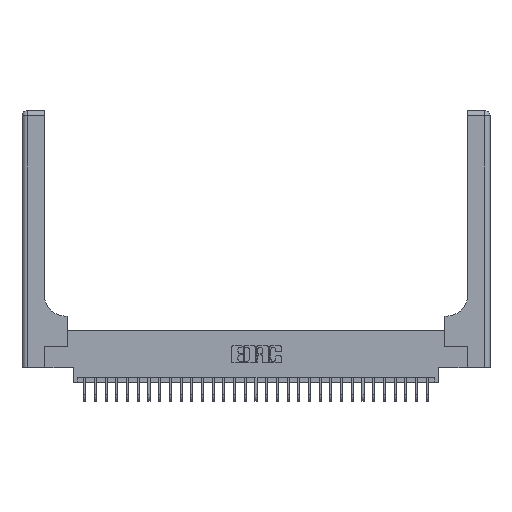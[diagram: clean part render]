
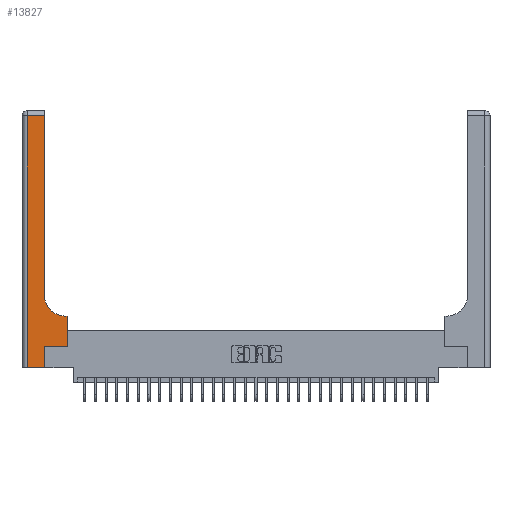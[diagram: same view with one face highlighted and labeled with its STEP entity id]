
A CAD part, top view. The second image highlights one B-rep face of the part: STEP entity #13827.
In plain terms, the highlighted planar face has unit normal (0, 0, 1).
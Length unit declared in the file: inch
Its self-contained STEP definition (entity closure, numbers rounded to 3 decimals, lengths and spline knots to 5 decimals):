
#315 = DIRECTION ( 'NONE',  ( 0., 1., 0. ) ) ;
#471 = CARTESIAN_POINT ( 'NONE',  ( 0.528, 0.25, 0.37 ) ) ;
#1172 = EDGE_CURVE ( 'NONE', #22529, #27195, #14642, .T. ) ;
#1348 = EDGE_CURVE ( 'NONE', #7076, #21148, #24732, .T. ) ;
#1525 = CARTESIAN_POINT ( 'NONE',  ( 0.06, 2.94, 0.37 ) ) ;
#1708 = CARTESIAN_POINT ( 'NONE',  ( 0.265, 0.25, 0.37 ) ) ;
#1849 = CARTESIAN_POINT ( 'NONE',  ( 0.265, 0.25, 0.37 ) ) ;
#2572 = VERTEX_POINT ( 'NONE', #21076 ) ;
#2679 = DIRECTION ( 'NONE',  ( 0., 0., -1. ) ) ;
#3170 = CARTESIAN_POINT ( 'NONE',  ( 0.06, 0., 0.37 ) ) ;
#3246 = AXIS2_PLACEMENT_3D ( 'NONE', #16298, #2679, #21384 ) ;
#4025 = EDGE_CURVE ( 'NONE', #10255, #10194, #4784, .T. ) ;
#4306 = ORIENTED_EDGE ( 'NONE', *, *, #1348, .T. ) ;
#4591 = EDGE_CURVE ( 'NONE', #10247, #22529, #27288, .T. ) ;
#4784 = LINE ( 'NONE', #16699, #14586 ) ;
#5008 = CARTESIAN_POINT ( 'NONE',  ( 0.265, 0., 0.37 ) ) ;
#5709 = DIRECTION ( 'NONE',  ( 1., 0., 0. ) ) ;
#5772 = CARTESIAN_POINT ( 'NONE',  ( 0.51, 0.6, 0.37 ) ) ;
#6225 = LINE ( 'NONE', #15553, #24726 ) ;
#7023 = ORIENTED_EDGE ( 'NONE', *, *, #20876, .T. ) ;
#7076 = VERTEX_POINT ( 'NONE', #27183 ) ;
#8366 = ORIENTED_EDGE ( 'NONE', *, *, #10621, .T. ) ;
#8431 = DIRECTION ( 'NONE',  ( 1., 0., 0. ) ) ;
#9112 = DIRECTION ( 'NONE',  ( -1., 0., 0. ) ) ;
#9415 = FACE_OUTER_BOUND ( 'NONE', #29696, .T. ) ;
#9507 = LINE ( 'NONE', #471, #24153 ) ;
#9653 = DIRECTION ( 'NONE',  ( -1., 0., 0. ) ) ;
#9687 = VECTOR ( 'NONE', #10799, 39.37008 ) ;
#10194 = VERTEX_POINT ( 'NONE', #5772 ) ;
#10247 = VERTEX_POINT ( 'NONE', #3170 ) ;
#10255 = VERTEX_POINT ( 'NONE', #29217 ) ;
#10621 = EDGE_CURVE ( 'NONE', #10194, #12486, #13497, .T. ) ;
#10799 = DIRECTION ( 'NONE',  ( 0., -1., 0. ) ) ;
#10882 = LINE ( 'NONE', #1708, #29936 ) ;
#10944 = CARTESIAN_POINT ( 'NONE',  ( 0.26, 0.85, 0.37 ) ) ;
#11467 = CARTESIAN_POINT ( 'NONE',  ( 0.265, 0., 0.37 ) ) ;
#12486 = VERTEX_POINT ( 'NONE', #10944 ) ;
#12857 = ORIENTED_EDGE ( 'NONE', *, *, #15804, .T. ) ;
#13141 = DIRECTION ( 'NONE',  ( 0., 0., -1. ) ) ;
#13228 = DIRECTION ( 'NONE',  ( -1., 0., 0. ) ) ;
#13292 = ORIENTED_EDGE ( 'NONE', *, *, #24489, .T. ) ;
#13402 = DIRECTION ( 'NONE',  ( 0., 1., 0. ) ) ;
#13497 = CIRCLE ( 'NONE', #3246, 0.25 ) ;
#13827 = ADVANCED_FACE ( 'NONE', ( #9415 ), #28128, .F. ) ;
#14586 = VECTOR ( 'NONE', #9653, 39.37008 ) ;
#14642 = LINE ( 'NONE', #5008, #27295 ) ;
#15553 = CARTESIAN_POINT ( 'NONE',  ( 0.26, 3., 0.37 ) ) ;
#15804 = EDGE_CURVE ( 'NONE', #27195, #2572, #10882, .T. ) ;
#16298 = CARTESIAN_POINT ( 'NONE',  ( 0.51, 0.85, 0.37 ) ) ;
#16699 = CARTESIAN_POINT ( 'NONE',  ( 0.26, 0.6, 0.37 ) ) ;
#17931 = EDGE_CURVE ( 'NONE', #21148, #10247, #29521, .T. ) ;
#18008 = VECTOR ( 'NONE', #8431, 39.37008 ) ;
#19139 = ORIENTED_EDGE ( 'NONE', *, *, #1172, .T. ) ;
#19397 = DIRECTION ( 'NONE',  ( 0., 1., 0. ) ) ;
#20308 = CARTESIAN_POINT ( 'NONE',  ( 0., 2.94, 0.37 ) ) ;
#20876 = EDGE_CURVE ( 'NONE', #2572, #10255, #9507, .T. ) ;
#21076 = CARTESIAN_POINT ( 'NONE',  ( 0.528, 0.25, 0.37 ) ) ;
#21148 = VERTEX_POINT ( 'NONE', #1525 ) ;
#21384 = DIRECTION ( 'NONE',  ( 1., 0., 0. ) ) ;
#21888 = ORIENTED_EDGE ( 'NONE', *, *, #4025, .T. ) ;
#22395 = CARTESIAN_POINT ( 'NONE',  ( 0., 0., 0.37 ) ) ;
#22479 = CARTESIAN_POINT ( 'NONE',  ( 0.06, 3., 0.37 ) ) ;
#22529 = VERTEX_POINT ( 'NONE', #11467 ) ;
#24153 = VECTOR ( 'NONE', #315, 39.37008 ) ;
#24287 = ORIENTED_EDGE ( 'NONE', *, *, #17931, .T. ) ;
#24489 = EDGE_CURVE ( 'NONE', #12486, #7076, #6225, .T. ) ;
#24726 = VECTOR ( 'NONE', #13402, 39.37008 ) ;
#24727 = AXIS2_PLACEMENT_3D ( 'NONE', #25826, #13141, #9112 ) ;
#24732 = LINE ( 'NONE', #20308, #28299 ) ;
#25826 = CARTESIAN_POINT ( 'NONE',  ( 0., 3., 0.37 ) ) ;
#27183 = CARTESIAN_POINT ( 'NONE',  ( 0.26, 2.94, 0.37 ) ) ;
#27195 = VERTEX_POINT ( 'NONE', #1849 ) ;
#27288 = LINE ( 'NONE', #22395, #18008 ) ;
#27295 = VECTOR ( 'NONE', #19397, 39.37008 ) ;
#28128 = PLANE ( 'NONE',  #24727 ) ;
#28299 = VECTOR ( 'NONE', #13228, 39.37008 ) ;
#29217 = CARTESIAN_POINT ( 'NONE',  ( 0.528, 0.6, 0.37 ) ) ;
#29521 = LINE ( 'NONE', #22479, #9687 ) ;
#29696 = EDGE_LOOP ( 'NONE', ( #13292, #4306, #24287, #29954, #19139, #12857, #7023, #21888, #8366 ) ) ;
#29936 = VECTOR ( 'NONE', #5709, 39.37008 ) ;
#29954 = ORIENTED_EDGE ( 'NONE', *, *, #4591, .T. ) ;
